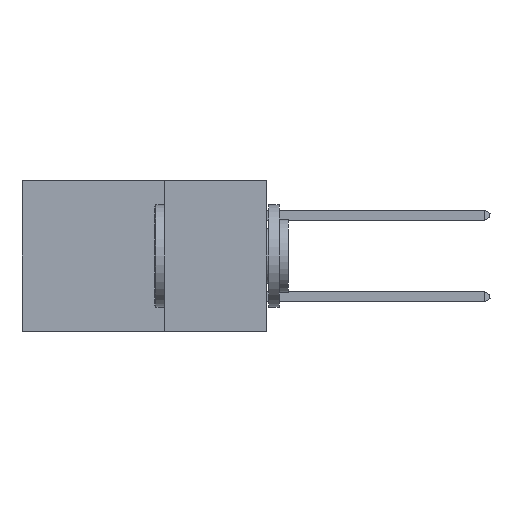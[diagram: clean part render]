
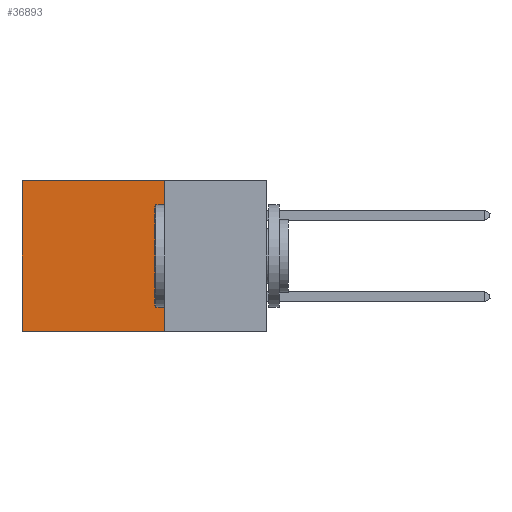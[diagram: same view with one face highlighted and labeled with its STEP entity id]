
A CAD part, left-side view. The second image highlights one B-rep face of the part: STEP entity #36893.
In plain terms, the highlighted planar face has unit normal (-1, 0, 0).
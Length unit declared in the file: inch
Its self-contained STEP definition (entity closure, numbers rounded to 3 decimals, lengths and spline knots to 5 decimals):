
#411 = CARTESIAN_POINT ( 'NONE',  ( 0.2875, 0.6, -0.37 ) ) ;
#511 = VECTOR ( 'NONE', #25524, 39.37008 ) ;
#2571 = CARTESIAN_POINT ( 'NONE',  ( 0.2875, 0.25, 0. ) ) ;
#3441 = VECTOR ( 'NONE', #37501, 39.37008 ) ;
#4029 = CARTESIAN_POINT ( 'NONE',  ( 0.2875, 0.6, 0. ) ) ;
#6932 = EDGE_CURVE ( 'NONE', #38891, #36317, #39408, .T. ) ;
#8443 = EDGE_CURVE ( 'NONE', #23104, #36317, #36736, .T. ) ;
#11342 = CARTESIAN_POINT ( 'NONE',  ( 0.2875, 0.25, -0.37 ) ) ;
#12054 = VERTEX_POINT ( 'NONE', #2571 ) ;
#13620 = EDGE_CURVE ( 'NONE', #12054, #23104, #19876, .T. ) ;
#13728 = LINE ( 'NONE', #39401, #32896 ) ;
#13883 = ORIENTED_EDGE ( 'NONE', *, *, #6932, .F. ) ;
#15891 = VECTOR ( 'NONE', #40412, 39.37008 ) ;
#16339 = CARTESIAN_POINT ( 'NONE',  ( 0.2875, 0.6, 0. ) ) ;
#19876 = LINE ( 'NONE', #37191, #3441 ) ;
#20779 = PLANE ( 'NONE',  #23728 ) ;
#20928 = DIRECTION ( 'NONE',  ( 0., 0., -1. ) ) ;
#23104 = VERTEX_POINT ( 'NONE', #4029 ) ;
#23728 = AXIS2_PLACEMENT_3D ( 'NONE', #38063, #24302, #20928 ) ;
#24302 = DIRECTION ( 'NONE',  ( 1., 0., 0. ) ) ;
#25198 = DIRECTION ( 'NONE',  ( 0., 0., -1. ) ) ;
#25524 = DIRECTION ( 'NONE',  ( 0., 1., 0. ) ) ;
#28325 = ORIENTED_EDGE ( 'NONE', *, *, #30011, .F. ) ;
#29346 = EDGE_LOOP ( 'NONE', ( #42592, #13883, #28325, #34946 ) ) ;
#30011 = EDGE_CURVE ( 'NONE', #12054, #38891, #13728, .T. ) ;
#32896 = VECTOR ( 'NONE', #25198, 39.37008 ) ;
#34946 = ORIENTED_EDGE ( 'NONE', *, *, #13620, .T. ) ;
#36317 = VERTEX_POINT ( 'NONE', #411 ) ;
#36736 = LINE ( 'NONE', #16339, #15891 ) ;
#36893 = ADVANCED_FACE ( 'NONE', ( #38133 ), #20779, .F. ) ;
#37191 = CARTESIAN_POINT ( 'NONE',  ( 0.2875, 0.25, 0. ) ) ;
#37501 = DIRECTION ( 'NONE',  ( 0., 1., 0. ) ) ;
#38063 = CARTESIAN_POINT ( 'NONE',  ( 0.2875, 0.25, 0. ) ) ;
#38133 = FACE_OUTER_BOUND ( 'NONE', #29346, .T. ) ;
#38891 = VERTEX_POINT ( 'NONE', #11342 ) ;
#39285 = CARTESIAN_POINT ( 'NONE',  ( 0.2875, 0.25, -0.37 ) ) ;
#39401 = CARTESIAN_POINT ( 'NONE',  ( 0.2875, 0.25, 0. ) ) ;
#39408 = LINE ( 'NONE', #39285, #511 ) ;
#40412 = DIRECTION ( 'NONE',  ( 0., 0., -1. ) ) ;
#42592 = ORIENTED_EDGE ( 'NONE', *, *, #8443, .T. ) ;
